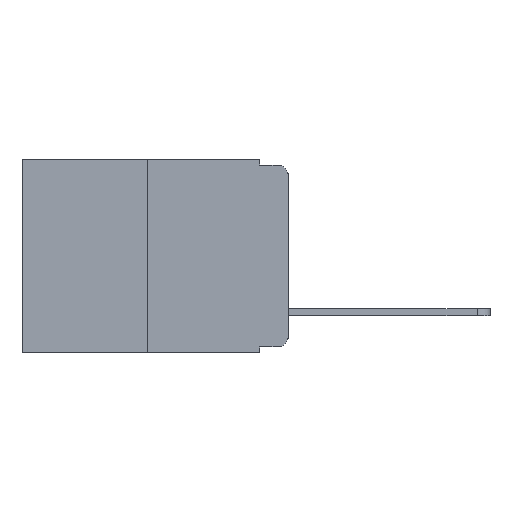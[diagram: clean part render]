
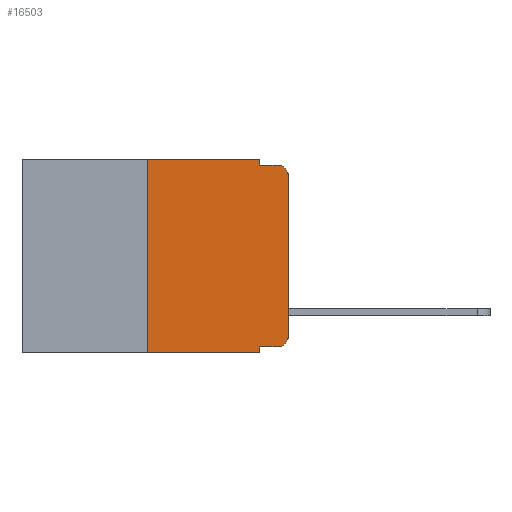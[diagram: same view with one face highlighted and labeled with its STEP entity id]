
A CAD part, left-side view. The second image highlights one B-rep face of the part: STEP entity #16503.
In plain terms, the highlighted planar face has unit normal (-1, 0, 0).
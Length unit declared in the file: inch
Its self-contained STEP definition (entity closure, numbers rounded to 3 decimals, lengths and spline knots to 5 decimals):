
#129 = VERTEX_POINT ( 'NONE', #18049 ) ;
#547 = LINE ( 'NONE', #1598, #16165 ) ;
#752 = VECTOR ( 'NONE', #6829, 39.37008 ) ;
#829 = DIRECTION ( 'NONE',  ( 0., -1., 0. ) ) ;
#860 = LINE ( 'NONE', #17766, #12738 ) ;
#896 = ORIENTED_EDGE ( 'NONE', *, *, #7060, .F. ) ;
#1598 = CARTESIAN_POINT ( 'NONE',  ( 0., 0.051, -0.01 ) ) ;
#1919 = VERTEX_POINT ( 'NONE', #2733 ) ;
#1944 = CARTESIAN_POINT ( 'NONE',  ( 0., 0.051, -0.343 ) ) ;
#1959 = VERTEX_POINT ( 'NONE', #13622 ) ;
#2088 = EDGE_LOOP ( 'NONE', ( #11897, #4563, #896, #5015, #9031, #9480, #16904, #9938, #17337, #10389 ) ) ;
#2372 = EDGE_CURVE ( 'NONE', #11258, #1919, #10465, .T. ) ;
#2446 = CARTESIAN_POINT ( 'NONE',  ( 0., 0., 0. ) ) ;
#2574 = AXIS2_PLACEMENT_3D ( 'NONE', #14706, #14671, #14686 ) ;
#2733 = CARTESIAN_POINT ( 'NONE',  ( 0., 0.02, -0.01 ) ) ;
#3055 = LINE ( 'NONE', #13891, #10960 ) ;
#3255 = VERTEX_POINT ( 'NONE', #7027 ) ;
#3267 = EDGE_CURVE ( 'NONE', #16063, #3255, #10428, .T. ) ;
#3505 = CARTESIAN_POINT ( 'NONE',  ( 0., 0.051, 0. ) ) ;
#3832 = CARTESIAN_POINT ( 'NONE',  ( 0., 0., -0.03 ) ) ;
#3917 = VERTEX_POINT ( 'NONE', #16345 ) ;
#4563 = ORIENTED_EDGE ( 'NONE', *, *, #2372, .T. ) ;
#4706 = VERTEX_POINT ( 'NONE', #10861 ) ;
#4736 = DIRECTION ( 'NONE',  ( 1., 0., 0. ) ) ;
#4872 = LINE ( 'NONE', #12577, #752 ) ;
#5015 = ORIENTED_EDGE ( 'NONE', *, *, #3267, .F. ) ;
#5531 = EDGE_CURVE ( 'NONE', #1959, #4706, #11458, .T. ) ;
#6015 = VECTOR ( 'NONE', #17381, 39.37008 ) ;
#6829 = DIRECTION ( 'NONE',  ( 0., -1., 0. ) ) ;
#7027 = CARTESIAN_POINT ( 'NONE',  ( 0., 0.051, -0.01 ) ) ;
#7060 = EDGE_CURVE ( 'NONE', #3255, #1919, #547, .T. ) ;
#7458 = EDGE_CURVE ( 'NONE', #4706, #11258, #9613, .T. ) ;
#8020 = DIRECTION ( 'NONE',  ( 0., 0., -1. ) ) ;
#8576 = EDGE_CURVE ( 'NONE', #129, #1959, #4872, .T. ) ;
#8595 = DIRECTION ( 'NONE',  ( 0., 0., 1. ) ) ;
#8824 = DIRECTION ( 'NONE',  ( -1., 0., 0. ) ) ;
#8858 = VECTOR ( 'NONE', #9971, 39.37008 ) ;
#8972 = EDGE_CURVE ( 'NONE', #17274, #16063, #15969, .T. ) ;
#8976 = VECTOR ( 'NONE', #829, 39.37008 ) ;
#9024 = CARTESIAN_POINT ( 'NONE',  ( 0., 0.02, -0.03 ) ) ;
#9031 = ORIENTED_EDGE ( 'NONE', *, *, #8972, .F. ) ;
#9480 = ORIENTED_EDGE ( 'NONE', *, *, #14199, .F. ) ;
#9541 = EDGE_CURVE ( 'NONE', #129, #11128, #3055, .T. ) ;
#9613 = LINE ( 'NONE', #2446, #12897 ) ;
#9765 = AXIS2_PLACEMENT_3D ( 'NONE', #17573, #4736, #14792 ) ;
#9938 = ORIENTED_EDGE ( 'NONE', *, *, #9541, .F. ) ;
#9941 = CARTESIAN_POINT ( 'NONE',  ( 0., 0.473, 0. ) ) ;
#9971 = DIRECTION ( 'NONE',  ( 0., -1., 0. ) ) ;
#10389 = ORIENTED_EDGE ( 'NONE', *, *, #5531, .T. ) ;
#10428 = LINE ( 'NONE', #18448, #6015 ) ;
#10465 = CIRCLE ( 'NONE', #10668, 0.02 ) ;
#10668 = AXIS2_PLACEMENT_3D ( 'NONE', #9024, #8824, #8020 ) ;
#10858 = DIRECTION ( 'NONE',  ( 0., 0., 1. ) ) ;
#10861 = CARTESIAN_POINT ( 'NONE',  ( 0., 0., -0.313 ) ) ;
#10960 = VECTOR ( 'NONE', #16735, 39.37008 ) ;
#11128 = VERTEX_POINT ( 'NONE', #1944 ) ;
#11258 = VERTEX_POINT ( 'NONE', #3832 ) ;
#11458 = CIRCLE ( 'NONE', #2574, 0.02 ) ;
#11897 = ORIENTED_EDGE ( 'NONE', *, *, #7458, .T. ) ;
#12577 = CARTESIAN_POINT ( 'NONE',  ( 0., 0.051, -0.333 ) ) ;
#12595 = LINE ( 'NONE', #15477, #8858 ) ;
#12738 = VECTOR ( 'NONE', #10858, 39.37008 ) ;
#12897 = VECTOR ( 'NONE', #8595, 39.37008 ) ;
#13378 = DIRECTION ( 'NONE',  ( 0., -1., 0. ) ) ;
#13411 = PLANE ( 'NONE',  #9765 ) ;
#13622 = CARTESIAN_POINT ( 'NONE',  ( 0., 0.02, -0.333 ) ) ;
#13891 = CARTESIAN_POINT ( 'NONE',  ( 0., 0.051, 0. ) ) ;
#14092 = FACE_OUTER_BOUND ( 'NONE', #2088, .T. ) ;
#14199 = EDGE_CURVE ( 'NONE', #3917, #17274, #860, .T. ) ;
#14579 = CARTESIAN_POINT ( 'NONE',  ( 0., 0.25, 0. ) ) ;
#14671 = DIRECTION ( 'NONE',  ( -1., 0., 0. ) ) ;
#14686 = DIRECTION ( 'NONE',  ( 0., 0., -1. ) ) ;
#14706 = CARTESIAN_POINT ( 'NONE',  ( 0., 0.02, -0.313 ) ) ;
#14792 = DIRECTION ( 'NONE',  ( 0., 0., -1. ) ) ;
#15477 = CARTESIAN_POINT ( 'NONE',  ( 0., 0.473, -0.343 ) ) ;
#15969 = LINE ( 'NONE', #9941, #8976 ) ;
#16063 = VERTEX_POINT ( 'NONE', #3505 ) ;
#16165 = VECTOR ( 'NONE', #13378, 39.37008 ) ;
#16345 = CARTESIAN_POINT ( 'NONE',  ( 0., 0.25, -0.343 ) ) ;
#16503 = ADVANCED_FACE ( 'NONE', ( #14092 ), #13411, .F. ) ;
#16735 = DIRECTION ( 'NONE',  ( 0., 0., -1. ) ) ;
#16784 = EDGE_CURVE ( 'NONE', #3917, #11128, #12595, .T. ) ;
#16904 = ORIENTED_EDGE ( 'NONE', *, *, #16784, .T. ) ;
#17274 = VERTEX_POINT ( 'NONE', #14579 ) ;
#17337 = ORIENTED_EDGE ( 'NONE', *, *, #8576, .T. ) ;
#17381 = DIRECTION ( 'NONE',  ( 0., 0., -1. ) ) ;
#17573 = CARTESIAN_POINT ( 'NONE',  ( 0., 0.473, 0. ) ) ;
#17766 = CARTESIAN_POINT ( 'NONE',  ( 0., 0.25, 0. ) ) ;
#18049 = CARTESIAN_POINT ( 'NONE',  ( 0., 0.051, -0.333 ) ) ;
#18448 = CARTESIAN_POINT ( 'NONE',  ( 0., 0.051, 0. ) ) ;
